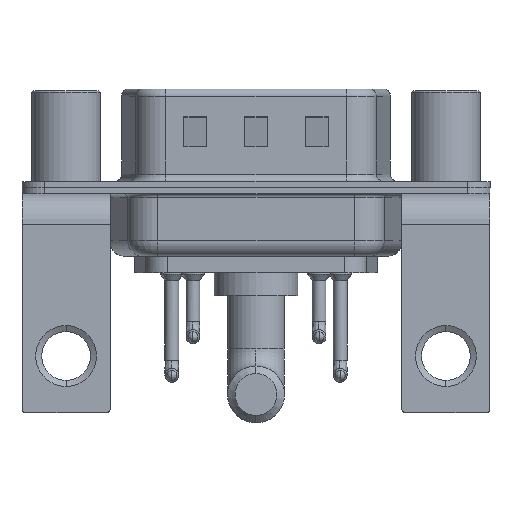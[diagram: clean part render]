
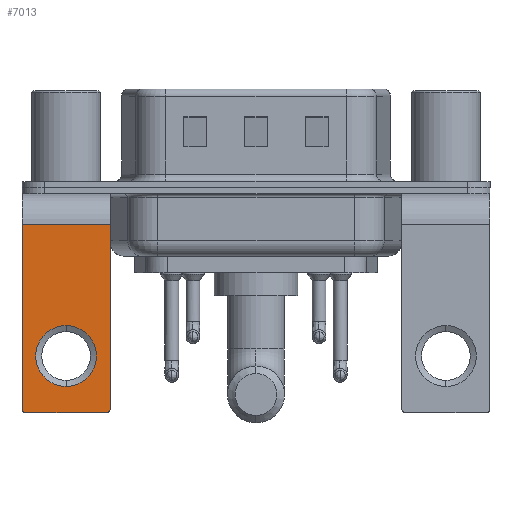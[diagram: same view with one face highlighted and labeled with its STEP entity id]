
A CAD part, front view. The second image highlights one B-rep face of the part: STEP entity #7013.
In plain terms, the highlighted planar face has unit normal (0, -1, 0).
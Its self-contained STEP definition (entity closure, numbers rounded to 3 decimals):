
#55 = CIRCLE ( 'NONE', #3976, 0.25 ) ;
#912 = VERTEX_POINT ( 'NONE', #21775 ) ;
#1330 = LINE ( 'NONE', #21336, #2366 ) ;
#1585 = VECTOR ( 'NONE', #10799, 1000. ) ;
#2187 = CARTESIAN_POINT ( 'NONE',  ( -2.65, -6.25, -14.55 ) ) ;
#2194 = EDGE_CURVE ( 'NONE', #21729, #16494, #20365, .T. ) ;
#2366 = VECTOR ( 'NONE', #2997, 1000. ) ;
#2451 = ORIENTED_EDGE ( 'NONE', *, *, #18959, .T. ) ;
#2633 = DIRECTION ( 'NONE',  ( 0., 0., 1. ) ) ;
#2997 = DIRECTION ( 'NONE',  ( 0., 0., -1. ) ) ;
#3266 = ORIENTED_EDGE ( 'NONE', *, *, #13609, .F. ) ;
#3976 = AXIS2_PLACEMENT_3D ( 'NONE', #2187, #8925, #16367 ) ;
#4153 = EDGE_LOOP ( 'NONE', ( #20414, #5246 ) ) ;
#4587 = CARTESIAN_POINT ( 'NONE',  ( 2.9, -6.25, -14.8 ) ) ;
#4802 = ORIENTED_EDGE ( 'NONE', *, *, #18146, .F. ) ;
#5246 = ORIENTED_EDGE ( 'NONE', *, *, #2194, .T. ) ;
#5294 = DIRECTION ( 'NONE',  ( 0., 1., 0. ) ) ;
#6311 = CARTESIAN_POINT ( 'NONE',  ( 2.9, -6.25, -14.55 ) ) ;
#6358 = CARTESIAN_POINT ( 'NONE',  ( 0., -6.25, -11.07 ) ) ;
#6715 = AXIS2_PLACEMENT_3D ( 'NONE', #13913, #5294, #7173 ) ;
#6745 = EDGE_CURVE ( 'NONE', #912, #21615, #12974, .T. ) ;
#6984 = EDGE_CURVE ( 'NONE', #16494, #21729, #21544, .T. ) ;
#6989 = CIRCLE ( 'NONE', #10129, 0.25 ) ;
#7013 = ADVANCED_FACE ( 'NONE', ( #9358, #9259 ), #12920, .F. ) ;
#7173 = DIRECTION ( 'NONE',  ( 0., 0., 1. ) ) ;
#7400 = CARTESIAN_POINT ( 'NONE',  ( -2.9, -6.25, -2.4 ) ) ;
#7467 = VECTOR ( 'NONE', #11914, 1000. ) ;
#7820 = EDGE_CURVE ( 'NONE', #16097, #18407, #55, .T. ) ;
#8705 = AXIS2_PLACEMENT_3D ( 'NONE', #6358, #13117, #12787 ) ;
#8925 = DIRECTION ( 'NONE',  ( 0., -1., 0. ) ) ;
#9259 = FACE_OUTER_BOUND ( 'NONE', #17987, .T. ) ;
#9344 = DIRECTION ( 'NONE',  ( 0., 0., 1. ) ) ;
#9358 = FACE_BOUND ( 'NONE', #4153, .T. ) ;
#9477 = DIRECTION ( 'NONE',  ( 0., 1., 0. ) ) ;
#10129 = AXIS2_PLACEMENT_3D ( 'NONE', #12477, #20861, #9344 ) ;
#10379 = ORIENTED_EDGE ( 'NONE', *, *, #7820, .T. ) ;
#10692 = LINE ( 'NONE', #7400, #1585 ) ;
#10799 = DIRECTION ( 'NONE',  ( 0., 0., -1. ) ) ;
#11322 = DIRECTION ( 'NONE',  ( -1., 0., 0. ) ) ;
#11436 = CARTESIAN_POINT ( 'NONE',  ( 2.65, -6.25, -14.8 ) ) ;
#11914 = DIRECTION ( 'NONE',  ( -1., 0., 0. ) ) ;
#12156 = VERTEX_POINT ( 'NONE', #6311 ) ;
#12352 = EDGE_CURVE ( 'NONE', #21615, #16097, #10692, .T. ) ;
#12477 = CARTESIAN_POINT ( 'NONE',  ( 2.65, -6.25, -14.55 ) ) ;
#12787 = DIRECTION ( 'NONE',  ( 0., 0., 1. ) ) ;
#12920 = PLANE ( 'NONE',  #20124 ) ;
#12974 = LINE ( 'NONE', #18446, #7467 ) ;
#13117 = DIRECTION ( 'NONE',  ( 0., 1., 0. ) ) ;
#13609 = EDGE_CURVE ( 'NONE', #20347, #18407, #19723, .T. ) ;
#13913 = CARTESIAN_POINT ( 'NONE',  ( 0., -6.25, -11.07 ) ) ;
#14964 = CARTESIAN_POINT ( 'NONE',  ( 0., -6.25, -13.07 ) ) ;
#15308 = CARTESIAN_POINT ( 'NONE',  ( -2.9, -6.25, -14.55 ) ) ;
#15363 = CARTESIAN_POINT ( 'NONE',  ( -2.65, -6.25, -14.8 ) ) ;
#16066 = VECTOR ( 'NONE', #11322, 1000. ) ;
#16097 = VERTEX_POINT ( 'NONE', #15308 ) ;
#16367 = DIRECTION ( 'NONE',  ( 0., 0., 1. ) ) ;
#16494 = VERTEX_POINT ( 'NONE', #14964 ) ;
#16768 = CARTESIAN_POINT ( 'NONE',  ( 0., -6.25, -9.07 ) ) ;
#17670 = CARTESIAN_POINT ( 'NONE',  ( 2.9, -6.25, -2.4 ) ) ;
#17987 = EDGE_LOOP ( 'NONE', ( #19927, #10379, #3266, #2451, #4802, #19270 ) ) ;
#18146 = EDGE_CURVE ( 'NONE', #912, #12156, #1330, .T. ) ;
#18407 = VERTEX_POINT ( 'NONE', #15363 ) ;
#18446 = CARTESIAN_POINT ( 'NONE',  ( 2.9, -6.25, -2.4 ) ) ;
#18959 = EDGE_CURVE ( 'NONE', #20347, #12156, #6989, .T. ) ;
#19270 = ORIENTED_EDGE ( 'NONE', *, *, #6745, .T. ) ;
#19723 = LINE ( 'NONE', #4587, #16066 ) ;
#19927 = ORIENTED_EDGE ( 'NONE', *, *, #12352, .T. ) ;
#20124 = AXIS2_PLACEMENT_3D ( 'NONE', #17670, #9477, #2633 ) ;
#20347 = VERTEX_POINT ( 'NONE', #11436 ) ;
#20365 = CIRCLE ( 'NONE', #8705, 2. ) ;
#20414 = ORIENTED_EDGE ( 'NONE', *, *, #6984, .T. ) ;
#20861 = DIRECTION ( 'NONE',  ( 0., -1., 0. ) ) ;
#21310 = CARTESIAN_POINT ( 'NONE',  ( -2.9, -6.25, -2.4 ) ) ;
#21336 = CARTESIAN_POINT ( 'NONE',  ( 2.9, -6.25, -2.4 ) ) ;
#21544 = CIRCLE ( 'NONE', #6715, 2. ) ;
#21615 = VERTEX_POINT ( 'NONE', #21310 ) ;
#21729 = VERTEX_POINT ( 'NONE', #16768 ) ;
#21775 = CARTESIAN_POINT ( 'NONE',  ( 2.9, -6.25, -2.4 ) ) ;
